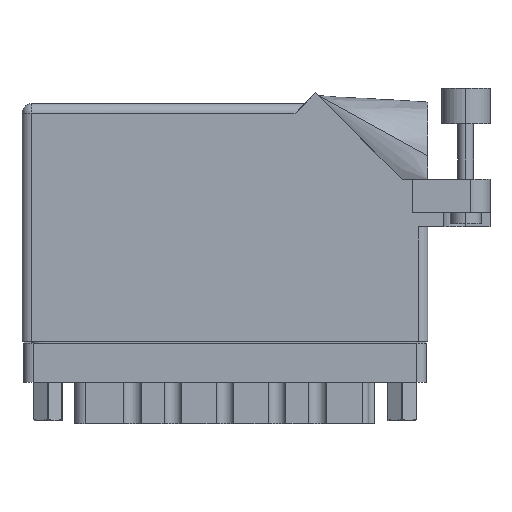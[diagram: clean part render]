
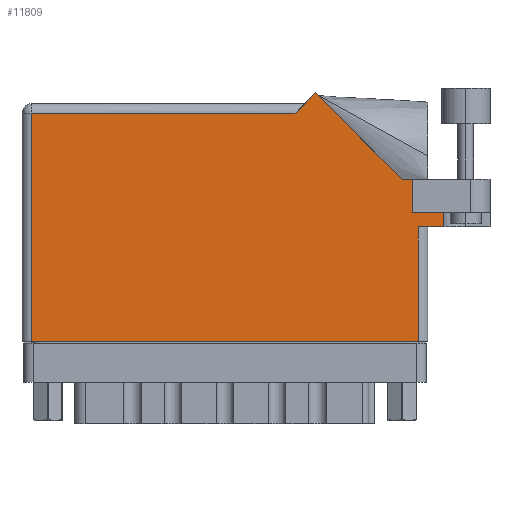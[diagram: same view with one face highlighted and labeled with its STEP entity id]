
A CAD part, front view. The second image highlights one B-rep face of the part: STEP entity #11809.
In plain terms, the highlighted face is planar.
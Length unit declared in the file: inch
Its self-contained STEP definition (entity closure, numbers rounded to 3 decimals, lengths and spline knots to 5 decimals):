
#649 = DIRECTION ( 'NONE',  ( -0.707, -0.707, 0. ) ) ;
#672 = VERTEX_POINT ( 'NONE', #10389 ) ;
#1887 = VECTOR ( 'NONE', #58547, 39.37008 ) ;
#3148 = ORIENTED_EDGE ( 'NONE', *, *, #57014, .T. ) ;
#3256 = DIRECTION ( 'NONE',  ( -1., 0., 0. ) ) ;
#3875 = ORIENTED_EDGE ( 'NONE', *, *, #27991, .T. ) ;
#4558 = CARTESIAN_POINT ( 'NONE',  ( 3.012, 1.044, 0. ) ) ;
#8155 = VERTEX_POINT ( 'NONE', #10057 ) ;
#8550 = DIRECTION ( 'NONE',  ( 0., 0., -1. ) ) ;
#10057 = CARTESIAN_POINT ( 'NONE',  ( 0.062, 0., 0. ) ) ;
#10389 = CARTESIAN_POINT ( 'NONE',  ( 2.512, 0.831, 0. ) ) ;
#11688 = EDGE_CURVE ( 'NONE', #31479, #40543, #53857, .T. ) ;
#11809 = ADVANCED_FACE ( 'NONE', ( #48573 ), #37438, .F. ) ;
#13669 = ORIENTED_EDGE ( 'NONE', *, *, #20570, .T. ) ;
#13874 = CARTESIAN_POINT ( 'NONE',  ( 2.7135, 0.737, 0. ) ) ;
#13922 = VECTOR ( 'NONE', #33580, 39.37008 ) ;
#14509 = VERTEX_POINT ( 'NONE', #26869 ) ;
#14729 = LINE ( 'NONE', #53870, #1887 ) ;
#15870 = ORIENTED_EDGE ( 'NONE', *, *, #17675, .T. ) ;
#17252 = CARTESIAN_POINT ( 'NONE',  ( 2.612, 0.737, 0. ) ) ;
#17561 = DIRECTION ( 'NONE',  ( 0., -1., 0. ) ) ;
#17675 = EDGE_CURVE ( 'NONE', #29887, #55321, #29668, .T. ) ;
#18107 = LINE ( 'NONE', #22009, #55138 ) ;
#18263 = CARTESIAN_POINT ( 'NONE',  ( 0., 1.53, 0. ) ) ;
#18300 = CARTESIAN_POINT ( 'NONE',  ( 1.757, 1.468, 0. ) ) ;
#19896 = CARTESIAN_POINT ( 'NONE',  ( 1.819, 1.53, 0. ) ) ;
#20570 = EDGE_CURVE ( 'NONE', #14509, #29887, #61938, .T. ) ;
#21616 = CARTESIAN_POINT ( 'NONE',  ( 0.062, 0., 0. ) ) ;
#22009 = CARTESIAN_POINT ( 'NONE',  ( 2.7135, 1.16177, 0. ) ) ;
#22100 = DIRECTION ( 'NONE',  ( -0.707, 0.707, 0. ) ) ;
#24094 = ORIENTED_EDGE ( 'NONE', *, *, #29314, .T. ) ;
#26642 = ORIENTED_EDGE ( 'NONE', *, *, #61260, .T. ) ;
#26869 = CARTESIAN_POINT ( 'NONE',  ( 2.44642, 1.044, 0. ) ) ;
#27057 = DIRECTION ( 'NONE',  ( 0., -1., 0. ) ) ;
#27991 = EDGE_CURVE ( 'NONE', #55321, #62388, #45781, .T. ) ;
#29044 = CARTESIAN_POINT ( 'NONE',  ( 2.7135, 0.831, 0. ) ) ;
#29226 = AXIS2_PLACEMENT_3D ( 'NONE', #18263, #8550, #3256 ) ;
#29314 = EDGE_CURVE ( 'NONE', #8155, #31479, #41056, .T. ) ;
#29668 = LINE ( 'NONE', #19896, #52367 ) ;
#29887 = VERTEX_POINT ( 'NONE', #47077 ) ;
#30205 = ORIENTED_EDGE ( 'NONE', *, *, #34570, .F. ) ;
#30834 = CARTESIAN_POINT ( 'NONE',  ( 2.55, 0., 0. ) ) ;
#31479 = VERTEX_POINT ( 'NONE', #30834 ) ;
#31999 = CARTESIAN_POINT ( 'NONE',  ( 2.44642, 1.044, 0. ) ) ;
#33580 = DIRECTION ( 'NONE',  ( 1., 0., 0. ) ) ;
#33810 = VERTEX_POINT ( 'NONE', #13874 ) ;
#34570 = EDGE_CURVE ( 'NONE', #672, #44841, #14729, .T. ) ;
#34892 = ORIENTED_EDGE ( 'NONE', *, *, #61165, .F. ) ;
#36714 = CARTESIAN_POINT ( 'NONE',  ( 2.55, 0.737, 0. ) ) ;
#37261 = DIRECTION ( 'NONE',  ( 1., 0., 0. ) ) ;
#37307 = CARTESIAN_POINT ( 'NONE',  ( 0., 1.468, 0. ) ) ;
#37438 = PLANE ( 'NONE',  #29226 ) ;
#38344 = EDGE_LOOP ( 'NONE', ( #24094, #45094, #55844, #34892, #30205, #43348, #3148, #13669, #15870, #3875, #26642 ) ) ;
#40543 = VERTEX_POINT ( 'NONE', #36714 ) ;
#40631 = CARTESIAN_POINT ( 'NONE',  ( 2.512, 0.831, 0. ) ) ;
#41056 = LINE ( 'NONE', #43096, #13922 ) ;
#43096 = CARTESIAN_POINT ( 'NONE',  ( 0., 0., 0. ) ) ;
#43348 = ORIENTED_EDGE ( 'NONE', *, *, #48028, .T. ) ;
#44233 = CARTESIAN_POINT ( 'NONE',  ( 2.512, 1.044, 0. ) ) ;
#44841 = VERTEX_POINT ( 'NONE', #29044 ) ;
#45094 = ORIENTED_EDGE ( 'NONE', *, *, #11688, .T. ) ;
#45278 = VECTOR ( 'NONE', #27057, 39.37008 ) ;
#45781 = LINE ( 'NONE', #37307, #47991 ) ;
#47067 = VECTOR ( 'NONE', #51420, 39.37008 ) ;
#47077 = CARTESIAN_POINT ( 'NONE',  ( 1.88971, 1.60071, 0. ) ) ;
#47858 = DIRECTION ( 'NONE',  ( -1., 0., 0. ) ) ;
#47991 = VECTOR ( 'NONE', #57002, 39.37008 ) ;
#48028 = EDGE_CURVE ( 'NONE', #672, #50324, #57609, .T. ) ;
#48324 = LINE ( 'NONE', #17252, #55127 ) ;
#48331 = VECTOR ( 'NONE', #22100, 39.37008 ) ;
#48573 = FACE_OUTER_BOUND ( 'NONE', #38344, .T. ) ;
#49211 = VECTOR ( 'NONE', #56087, 39.37008 ) ;
#49968 = CARTESIAN_POINT ( 'NONE',  ( 0.062, 1.468, 0. ) ) ;
#50073 = EDGE_CURVE ( 'NONE', #40543, #33810, #48324, .T. ) ;
#50324 = VERTEX_POINT ( 'NONE', #44233 ) ;
#51074 = LINE ( 'NONE', #4558, #59314 ) ;
#51420 = DIRECTION ( 'NONE',  ( 0., 1., 0. ) ) ;
#52367 = VECTOR ( 'NONE', #649, 39.37008 ) ;
#53857 = LINE ( 'NONE', #60532, #47067 ) ;
#53870 = CARTESIAN_POINT ( 'NONE',  ( 2.512, 0.831, 0. ) ) ;
#55127 = VECTOR ( 'NONE', #37261, 39.37008 ) ;
#55138 = VECTOR ( 'NONE', #17561, 39.37008 ) ;
#55321 = VERTEX_POINT ( 'NONE', #18300 ) ;
#55844 = ORIENTED_EDGE ( 'NONE', *, *, #50073, .T. ) ;
#56087 = DIRECTION ( 'NONE',  ( 0., 1., 0. ) ) ;
#56592 = LINE ( 'NONE', #21616, #45278 ) ;
#57002 = DIRECTION ( 'NONE',  ( -1., 0., 0. ) ) ;
#57014 = EDGE_CURVE ( 'NONE', #50324, #14509, #51074, .T. ) ;
#57609 = LINE ( 'NONE', #40631, #49211 ) ;
#58547 = DIRECTION ( 'NONE',  ( 1., 0., 0. ) ) ;
#59314 = VECTOR ( 'NONE', #47858, 39.37008 ) ;
#60532 = CARTESIAN_POINT ( 'NONE',  ( 2.55, 0.737, 0. ) ) ;
#61165 = EDGE_CURVE ( 'NONE', #44841, #33810, #18107, .T. ) ;
#61260 = EDGE_CURVE ( 'NONE', #62388, #8155, #56592, .T. ) ;
#61938 = LINE ( 'NONE', #31999, #48331 ) ;
#62388 = VERTEX_POINT ( 'NONE', #49968 ) ;
